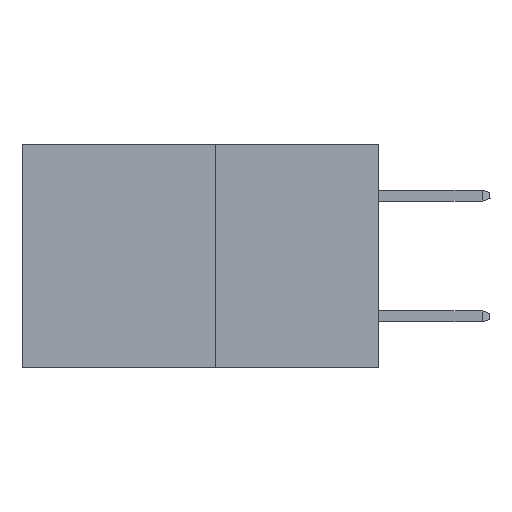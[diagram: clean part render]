
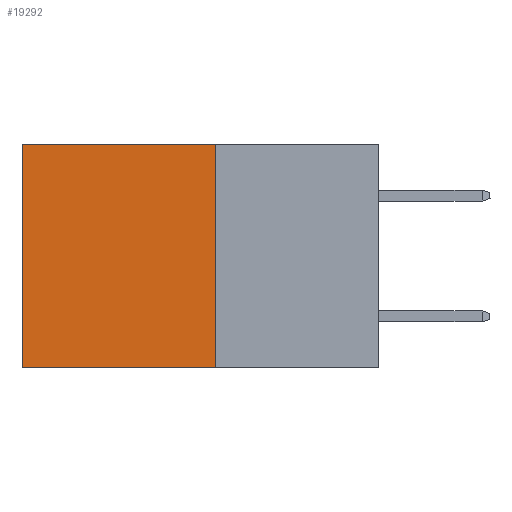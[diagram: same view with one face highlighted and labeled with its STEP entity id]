
A CAD part, left-side view. The second image highlights one B-rep face of the part: STEP entity #19292.
In plain terms, the highlighted planar face has unit normal (-1, 0, 0).
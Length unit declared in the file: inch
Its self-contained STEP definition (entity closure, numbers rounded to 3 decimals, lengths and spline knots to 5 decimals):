
#496 = PLANE ( 'NONE',  #23403 ) ;
#1103 = VERTEX_POINT ( 'NONE', #7854 ) ;
#1589 = DIRECTION ( 'NONE',  ( 0., 1., 0. ) ) ;
#1943 = CARTESIAN_POINT ( 'NONE',  ( 0.277, 0.27, 0. ) ) ;
#2978 = LINE ( 'NONE', #10515, #8085 ) ;
#3844 = DIRECTION ( 'NONE',  ( 0., 0., -1. ) ) ;
#4964 = DIRECTION ( 'NONE',  ( 0., 0., -1. ) ) ;
#6305 = EDGE_CURVE ( 'NONE', #1103, #19174, #24848, .T. ) ;
#6314 = ORIENTED_EDGE ( 'NONE', *, *, #6305, .T. ) ;
#7088 = VECTOR ( 'NONE', #1589, 39.37008 ) ;
#7566 = EDGE_CURVE ( 'NONE', #22925, #23150, #21802, .T. ) ;
#7854 = CARTESIAN_POINT ( 'NONE',  ( 0.277, 0.59, 0. ) ) ;
#8085 = VECTOR ( 'NONE', #27406, 39.37008 ) ;
#10241 = EDGE_CURVE ( 'NONE', #23150, #19174, #10762, .T. ) ;
#10325 = EDGE_CURVE ( 'NONE', #22925, #1103, #2978, .T. ) ;
#10515 = CARTESIAN_POINT ( 'NONE',  ( 0.277, 0.27, 0. ) ) ;
#10762 = LINE ( 'NONE', #22906, #7088 ) ;
#10993 = ORIENTED_EDGE ( 'NONE', *, *, #10241, .F. ) ;
#12764 = ORIENTED_EDGE ( 'NONE', *, *, #10325, .T. ) ;
#13044 = CARTESIAN_POINT ( 'NONE',  ( 0.277, 0.59, -0.37 ) ) ;
#13638 = VECTOR ( 'NONE', #15189, 39.37008 ) ;
#14565 = CARTESIAN_POINT ( 'NONE',  ( 0.277, 0.27, -0.37 ) ) ;
#15189 = DIRECTION ( 'NONE',  ( 0., 0., -1. ) ) ;
#15454 = FACE_OUTER_BOUND ( 'NONE', #24253, .T. ) ;
#15624 = CARTESIAN_POINT ( 'NONE',  ( 0.277, 0.27, -0.37 ) ) ;
#17275 = CARTESIAN_POINT ( 'NONE',  ( 0.277, 0.59, -0.37 ) ) ;
#17737 = DIRECTION ( 'NONE',  ( 1., 0., 0. ) ) ;
#19174 = VERTEX_POINT ( 'NONE', #17275 ) ;
#19292 = ADVANCED_FACE ( 'NONE', ( #15454 ), #496, .F. ) ;
#21802 = LINE ( 'NONE', #14565, #26093 ) ;
#21867 = CARTESIAN_POINT ( 'NONE',  ( 0.277, 0.27, -0.37 ) ) ;
#22492 = ORIENTED_EDGE ( 'NONE', *, *, #7566, .F. ) ;
#22906 = CARTESIAN_POINT ( 'NONE',  ( 0.277, 0.27, -0.37 ) ) ;
#22925 = VERTEX_POINT ( 'NONE', #1943 ) ;
#23150 = VERTEX_POINT ( 'NONE', #21867 ) ;
#23403 = AXIS2_PLACEMENT_3D ( 'NONE', #15624, #17737, #4964 ) ;
#24253 = EDGE_LOOP ( 'NONE', ( #6314, #10993, #22492, #12764 ) ) ;
#24848 = LINE ( 'NONE', #13044, #13638 ) ;
#26093 = VECTOR ( 'NONE', #3844, 39.37008 ) ;
#27406 = DIRECTION ( 'NONE',  ( 0., 1., 0. ) ) ;
